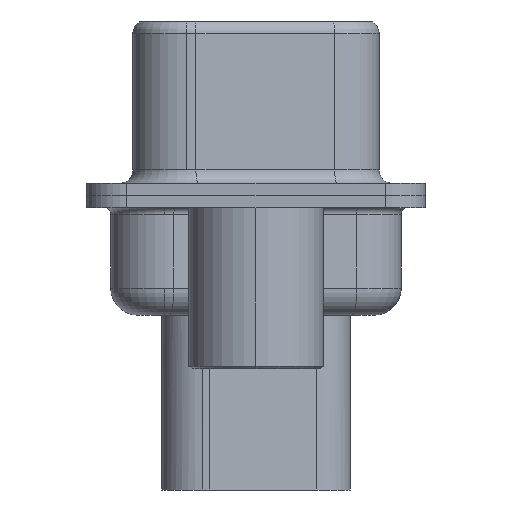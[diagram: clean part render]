
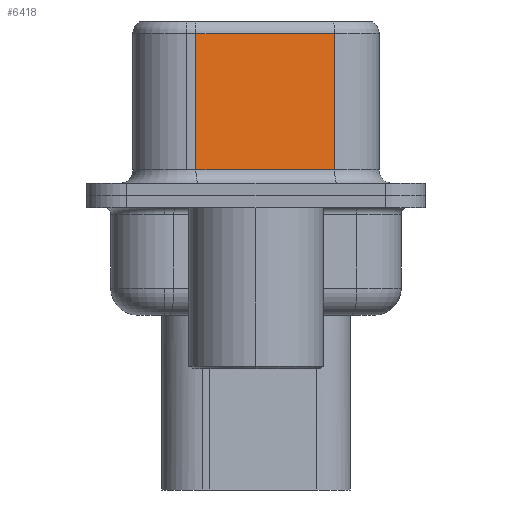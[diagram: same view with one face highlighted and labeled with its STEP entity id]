
A CAD part, left-side view. The second image highlights one B-rep face of the part: STEP entity #6418.
In plain terms, the highlighted planar face has unit normal (-0.985, -0.174, 0).
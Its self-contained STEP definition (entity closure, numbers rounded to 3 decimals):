
#405 = ORIENTED_EDGE ( 'NONE', *, *, #12175, .T. ) ;
#510 = CARTESIAN_POINT ( 'NONE',  ( 4.575, -2.927, 6.02 ) ) ;
#605 = DIRECTION ( 'NONE',  ( -0.174, 0.985, 0. ) ) ;
#878 = DIRECTION ( 'NONE',  ( 0., 0., -1. ) ) ;
#1716 = CARTESIAN_POINT ( 'NONE',  ( 3.665, 2.233, 0.95 ) ) ;
#2345 = VECTOR ( 'NONE', #878, 1000. ) ;
#2528 = EDGE_CURVE ( 'NONE', #5156, #8337, #7784, .T. ) ;
#2807 = AXIS2_PLACEMENT_3D ( 'NONE', #6423, #6493, #605 ) ;
#2872 = LINE ( 'NONE', #13645, #5931 ) ;
#3838 = VECTOR ( 'NONE', #13835, 1000. ) ;
#5156 = VERTEX_POINT ( 'NONE', #510 ) ;
#5931 = VECTOR ( 'NONE', #7670, 1000. ) ;
#6233 = CARTESIAN_POINT ( 'NONE',  ( 4.575, -2.927, 0.95 ) ) ;
#6418 = ADVANCED_FACE ( 'NONE', ( #8656 ), #12142, .F. ) ;
#6423 = CARTESIAN_POINT ( 'NONE',  ( 4.575, -2.927, 6.52 ) ) ;
#6493 = DIRECTION ( 'NONE',  ( 0.985, 0.174, 0. ) ) ;
#7302 = VERTEX_POINT ( 'NONE', #12558 ) ;
#7670 = DIRECTION ( 'NONE',  ( -0.174, 0.985, 0. ) ) ;
#7784 = LINE ( 'NONE', #8793, #13872 ) ;
#7925 = CARTESIAN_POINT ( 'NONE',  ( 3.665, 2.233, 6.52 ) ) ;
#8088 = CARTESIAN_POINT ( 'NONE',  ( 4.575, -2.927, 0.95 ) ) ;
#8337 = VERTEX_POINT ( 'NONE', #6233 ) ;
#8501 = EDGE_CURVE ( 'NONE', #10311, #8337, #11421, .T. ) ;
#8656 = FACE_OUTER_BOUND ( 'NONE', #9934, .T. ) ;
#8690 = ORIENTED_EDGE ( 'NONE', *, *, #2528, .F. ) ;
#8793 = CARTESIAN_POINT ( 'NONE',  ( 4.575, -2.927, 6.52 ) ) ;
#9934 = EDGE_LOOP ( 'NONE', ( #8690, #405, #10649, #13925 ) ) ;
#10311 = VERTEX_POINT ( 'NONE', #1716 ) ;
#10649 = ORIENTED_EDGE ( 'NONE', *, *, #14030, .T. ) ;
#11421 = LINE ( 'NONE', #8088, #3838 ) ;
#11497 = LINE ( 'NONE', #7925, #2345 ) ;
#12142 = PLANE ( 'NONE',  #2807 ) ;
#12175 = EDGE_CURVE ( 'NONE', #5156, #7302, #2872, .T. ) ;
#12558 = CARTESIAN_POINT ( 'NONE',  ( 3.665, 2.233, 6.02 ) ) ;
#13645 = CARTESIAN_POINT ( 'NONE',  ( 4.575, -2.927, 6.02 ) ) ;
#13835 = DIRECTION ( 'NONE',  ( 0.174, -0.985, 0. ) ) ;
#13872 = VECTOR ( 'NONE', #14533, 1000. ) ;
#13925 = ORIENTED_EDGE ( 'NONE', *, *, #8501, .T. ) ;
#14030 = EDGE_CURVE ( 'NONE', #7302, #10311, #11497, .T. ) ;
#14533 = DIRECTION ( 'NONE',  ( 0., 0., -1. ) ) ;
